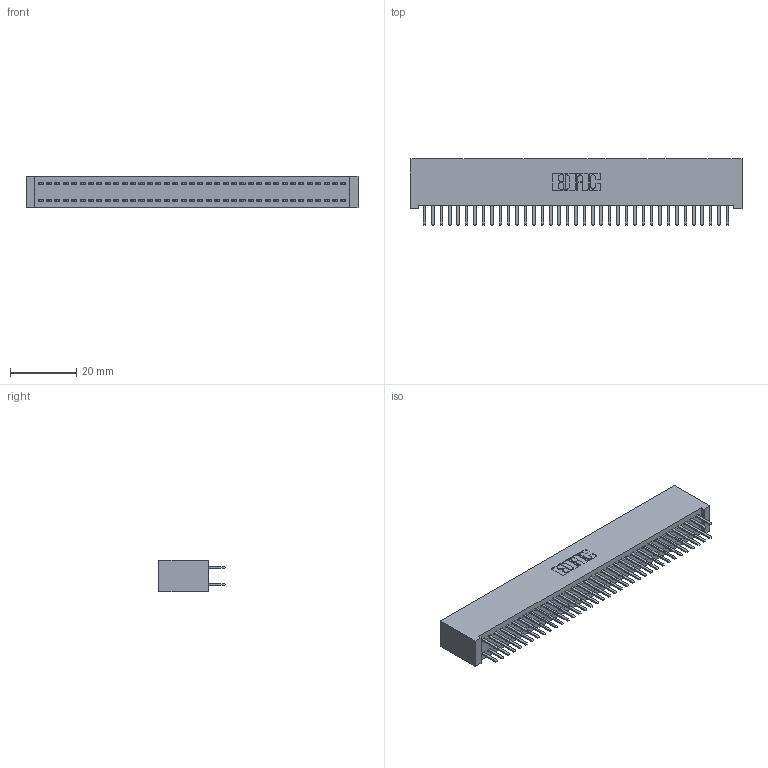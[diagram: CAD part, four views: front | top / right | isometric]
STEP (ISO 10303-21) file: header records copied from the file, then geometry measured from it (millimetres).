
FILE_DESCRIPTION (( 'STEP AP203' ), '1' );
FILE_NAME ('342-074-520-201.STEP', '2019-10-03T17:01:25', ( '' ), ( '' ), 'SwSTEP 2.0', 'SolidWorks 2016', '' );
FILE_SCHEMA (( 'CONFIG_CONTROL_DESIGN' ));
Length unit declared in the file: inch
Products named in the file (3): 342 Part_Lugless; 345-292-001_345-293-120; 342-074-520-201
Assembly tree (75 placements, depth 2):
  342-074-520-201
    342 Part_Lugless
    345-292-001_345-293-120  x74
Bounding box: 100.23 x 20.02 x 9.4 mm (x, y, z)
Volume: 9388.8 mm3; surface area: 15528.9 mm2
Topology: 75 solids, 75 shells, 4246 faces, 12337 edges, 8026 vertices
Faces by surface type: plane 2874, cylinder 1372
Entity records: 24155 total; most frequent: CARTESIAN_POINT 4018, ORIENTED_EDGE 3942, DIRECTION 3423, EDGE_CURVE 1971, VECTOR 1847, LINE 1847, VERTEX_POINT 1310, AXIS2_PLACEMENT_3D 788
